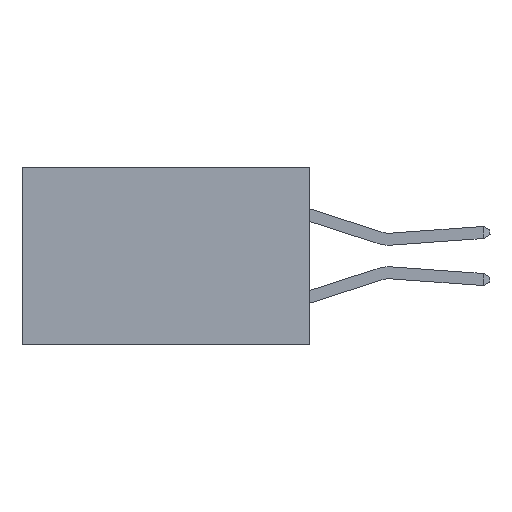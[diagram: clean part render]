
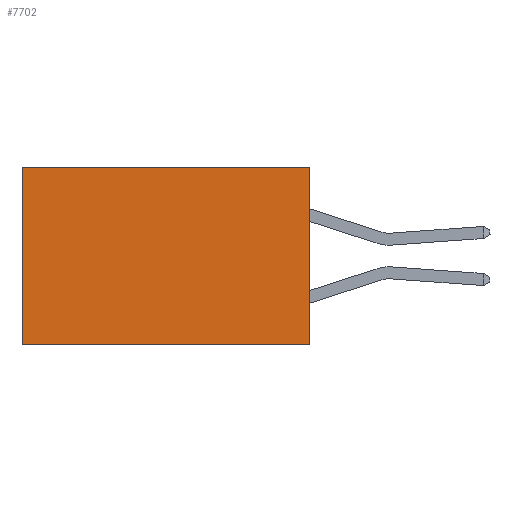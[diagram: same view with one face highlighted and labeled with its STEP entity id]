
A CAD part, left-side view. The second image highlights one B-rep face of the part: STEP entity #7702.
In plain terms, the highlighted planar face has unit normal (-1, 0, 0).
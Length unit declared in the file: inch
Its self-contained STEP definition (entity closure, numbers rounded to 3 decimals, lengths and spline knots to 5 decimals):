
#775 = DIRECTION ( 'NONE',  ( 0., 1., 0. ) ) ;
#973 = EDGE_LOOP ( 'NONE', ( #4958, #5224, #1807, #4775 ) ) ;
#1054 = EDGE_CURVE ( 'NONE', #1480, #1142, #4054, .T. ) ;
#1142 = VERTEX_POINT ( 'NONE', #5180 ) ;
#1480 = VERTEX_POINT ( 'NONE', #4611 ) ;
#1549 = VERTEX_POINT ( 'NONE', #6972 ) ;
#1807 = ORIENTED_EDGE ( 'NONE', *, *, #3193, .F. ) ;
#1928 = CARTESIAN_POINT ( 'NONE',  ( 0.298, 0., -0.37 ) ) ;
#2220 = VECTOR ( 'NONE', #3647, 39.37008 ) ;
#2676 = EDGE_CURVE ( 'NONE', #1549, #1480, #4367, .T. ) ;
#2730 = VECTOR ( 'NONE', #775, 39.37008 ) ;
#2938 = PLANE ( 'NONE',  #4792 ) ;
#3031 = DIRECTION ( 'NONE',  ( 0., 0., -1. ) ) ;
#3193 = EDGE_CURVE ( 'NONE', #1549, #6928, #7382, .T. ) ;
#3647 = DIRECTION ( 'NONE',  ( 0., 1., 0. ) ) ;
#3680 = DIRECTION ( 'NONE',  ( 0., 0., -1. ) ) ;
#4054 = LINE ( 'NONE', #7414, #8862 ) ;
#4367 = LINE ( 'NONE', #6312, #2220 ) ;
#4402 = CARTESIAN_POINT ( 'NONE',  ( 0.298, 0., -0.37 ) ) ;
#4611 = CARTESIAN_POINT ( 'NONE',  ( 0.298, 0.6, 0. ) ) ;
#4775 = ORIENTED_EDGE ( 'NONE', *, *, #2676, .T. ) ;
#4792 = AXIS2_PLACEMENT_3D ( 'NONE', #5077, #7825, #3680 ) ;
#4958 = ORIENTED_EDGE ( 'NONE', *, *, #1054, .T. ) ;
#5077 = CARTESIAN_POINT ( 'NONE',  ( 0.298, 0., 0. ) ) ;
#5180 = CARTESIAN_POINT ( 'NONE',  ( 0.298, 0.6, -0.37 ) ) ;
#5224 = ORIENTED_EDGE ( 'NONE', *, *, #7210, .F. ) ;
#6268 = LINE ( 'NONE', #4402, #2730 ) ;
#6312 = CARTESIAN_POINT ( 'NONE',  ( 0.298, 0., 0. ) ) ;
#6928 = VERTEX_POINT ( 'NONE', #1928 ) ;
#6972 = CARTESIAN_POINT ( 'NONE',  ( 0.298, 0., 0. ) ) ;
#7086 = CARTESIAN_POINT ( 'NONE',  ( 0.298, 0., 0. ) ) ;
#7172 = VECTOR ( 'NONE', #3031, 39.37008 ) ;
#7210 = EDGE_CURVE ( 'NONE', #6928, #1142, #6268, .T. ) ;
#7382 = LINE ( 'NONE', #7086, #7172 ) ;
#7414 = CARTESIAN_POINT ( 'NONE',  ( 0.298, 0.6, 0. ) ) ;
#7702 = ADVANCED_FACE ( 'NONE', ( #8989 ), #2938, .F. ) ;
#7811 = DIRECTION ( 'NONE',  ( 0., 0., -1. ) ) ;
#7825 = DIRECTION ( 'NONE',  ( 1., 0., 0. ) ) ;
#8862 = VECTOR ( 'NONE', #7811, 39.37008 ) ;
#8989 = FACE_OUTER_BOUND ( 'NONE', #973, .T. ) ;
